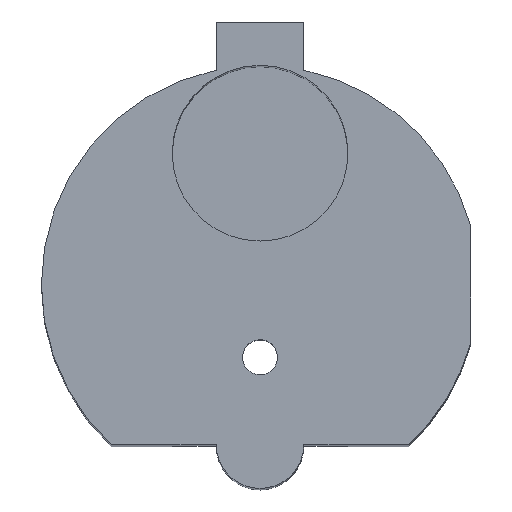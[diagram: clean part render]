
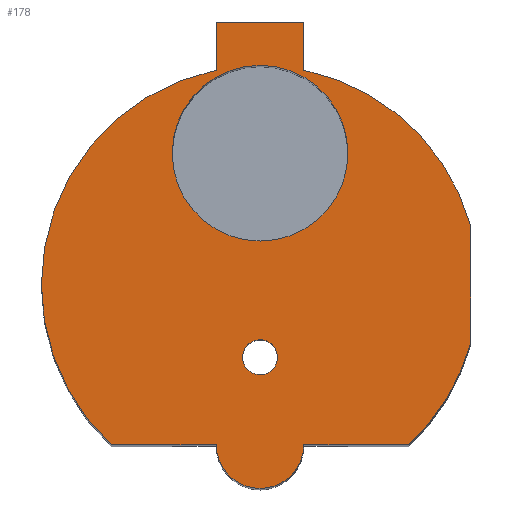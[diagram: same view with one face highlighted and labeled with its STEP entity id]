
A CAD part, top view. The second image highlights one B-rep face of the part: STEP entity #178.
In plain terms, the highlighted planar face has unit normal (0, 0, 1).
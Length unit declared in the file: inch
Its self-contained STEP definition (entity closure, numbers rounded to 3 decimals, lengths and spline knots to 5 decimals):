
#7 = AXIS2_PLACEMENT_3D ( 'NONE', #684, #1047, #1140 ) ;
#21 = AXIS2_PLACEMENT_3D ( 'NONE', #965, #514, #694 ) ;
#22 = VERTEX_POINT ( 'NONE', #44 ) ;
#27 = CARTESIAN_POINT ( 'NONE',  ( -0.15, 0.9, 2.9 ) ) ;
#42 = ORIENTED_EDGE ( 'NONE', *, *, #1071, .T. ) ;
#43 = CIRCLE ( 'NONE', #7, 0.75 ) ;
#44 = CARTESIAN_POINT ( 'NONE',  ( -0.30131, 0.45, 2.9 ) ) ;
#47 = ORIENTED_EDGE ( 'NONE', *, *, #1027, .F. ) ;
#55 = DIRECTION ( 'NONE',  ( 0., 0., 1. ) ) ;
#58 = PLANE ( 'NONE',  #457 ) ;
#68 = AXIS2_PLACEMENT_3D ( 'NONE', #913, #550, #823 ) ;
#70 = DIRECTION ( 'NONE',  ( 0., 1., 0. ) ) ;
#90 = ORIENTED_EDGE ( 'NONE', *, *, #865, .F. ) ;
#91 = VERTEX_POINT ( 'NONE', #329 ) ;
#103 = VERTEX_POINT ( 'NONE', #1134 ) ;
#105 = ORIENTED_EDGE ( 'NONE', *, *, #306, .F. ) ;
#108 = CARTESIAN_POINT ( 'NONE',  ( 0., -0.55, 2.9 ) ) ;
#112 = CIRCLE ( 'NONE', #620, 0.15 ) ;
#129 = AXIS2_PLACEMENT_3D ( 'NONE', #612, #55, #177 ) ;
#148 = DIRECTION ( 'NONE',  ( 0., -1., 0. ) ) ;
#177 = DIRECTION ( 'NONE',  ( 1., 0., 0. ) ) ;
#178 = ADVANCED_FACE ( 'NONE', ( #1092, #727, #943 ), #58, .T. ) ;
#201 = EDGE_CURVE ( 'NONE', #103, #91, #1144, .T. ) ;
#207 = VERTEX_POINT ( 'NONE', #982 ) ;
#211 = CARTESIAN_POINT ( 'NONE',  ( 0., 0.9, 2.9 ) ) ;
#223 = VERTEX_POINT ( 'NONE', #1039 ) ;
#229 = CARTESIAN_POINT ( 'NONE',  ( -0.15, 0., 2.9 ) ) ;
#235 = CARTESIAN_POINT ( 'NONE',  ( 0., -0.55, 2.9 ) ) ;
#255 = DIRECTION ( 'NONE',  ( 0., 0., -1. ) ) ;
#260 = EDGE_CURVE ( 'NONE', #561, #962, #885, .T. ) ;
#279 = VERTEX_POINT ( 'NONE', #798 ) ;
#304 = VERTEX_POINT ( 'NONE', #444 ) ;
#305 = CARTESIAN_POINT ( 'NONE',  ( -0.15, 0.73485, 2.9 ) ) ;
#306 = EDGE_CURVE ( 'NONE', #223, #22, #410, .T. ) ;
#310 = ORIENTED_EDGE ( 'NONE', *, *, #964, .T. ) ;
#312 = DIRECTION ( 'NONE',  ( 1., 0., 0. ) ) ;
#329 = CARTESIAN_POINT ( 'NONE',  ( -0.06, -0.25, 2.9 ) ) ;
#333 = LINE ( 'NONE', #563, #818 ) ;
#336 = LINE ( 'NONE', #526, #480 ) ;
#362 = DIRECTION ( 'NONE',  ( 1., 0., 0. ) ) ;
#374 = ORIENTED_EDGE ( 'NONE', *, *, #1106, .T. ) ;
#382 = CIRCLE ( 'NONE', #1146, 0.30131 ) ;
#410 = CIRCLE ( 'NONE', #961, 0.30131 ) ;
#424 = CIRCLE ( 'NONE', #1013, 0.06 ) ;
#425 = EDGE_CURVE ( 'NONE', #490, #207, #867, .T. ) ;
#440 = DIRECTION ( 'NONE',  ( 1., 0., 0. ) ) ;
#444 = CARTESIAN_POINT ( 'NONE',  ( -0.5099, -0.55, 2.9 ) ) ;
#446 = VECTOR ( 'NONE', #882, 39.37008 ) ;
#452 = CARTESIAN_POINT ( 'NONE',  ( 0., 0.45, 2.9 ) ) ;
#456 = DIRECTION ( 'NONE',  ( 0., 0., 1. ) ) ;
#457 = AXIS2_PLACEMENT_3D ( 'NONE', #975, #628, #440 ) ;
#478 = LINE ( 'NONE', #229, #1112 ) ;
#480 = VECTOR ( 'NONE', #70, 39.37008 ) ;
#490 = VERTEX_POINT ( 'NONE', #27 ) ;
#512 = DIRECTION ( 'NONE',  ( 1., 0., 0. ) ) ;
#514 = DIRECTION ( 'NONE',  ( 0., 0., 1. ) ) ;
#520 = LINE ( 'NONE', #108, #739 ) ;
#526 = CARTESIAN_POINT ( 'NONE',  ( 0.7222, 0., 2.9 ) ) ;
#533 = ORIENTED_EDGE ( 'NONE', *, *, #574, .T. ) ;
#539 = DIRECTION ( 'NONE',  ( 0., 0., 1. ) ) ;
#542 = CARTESIAN_POINT ( 'NONE',  ( 0.5099, -0.55, 2.9 ) ) ;
#550 = DIRECTION ( 'NONE',  ( 0., 0., -1. ) ) ;
#561 = VERTEX_POINT ( 'NONE', #542 ) ;
#563 = CARTESIAN_POINT ( 'NONE',  ( 0.15, 0., 2.9 ) ) ;
#573 = CARTESIAN_POINT ( 'NONE',  ( -0.15, -0.55, 2.9 ) ) ;
#574 = EDGE_CURVE ( 'NONE', #962, #747, #336, .T. ) ;
#576 = AXIS2_PLACEMENT_3D ( 'NONE', #980, #714, #721 ) ;
#592 = ORIENTED_EDGE ( 'NONE', *, *, #951, .T. ) ;
#594 = EDGE_CURVE ( 'NONE', #561, #920, #787, .T. ) ;
#612 = CARTESIAN_POINT ( 'NONE',  ( 0., 0., 2.9 ) ) ;
#620 = AXIS2_PLACEMENT_3D ( 'NONE', #235, #769, #512 ) ;
#628 = DIRECTION ( 'NONE',  ( 0., 0., 1. ) ) ;
#640 = VERTEX_POINT ( 'NONE', #1056 ) ;
#643 = CARTESIAN_POINT ( 'NONE',  ( 0.7222, 0.2023, 2.9 ) ) ;
#644 = ORIENTED_EDGE ( 'NONE', *, *, #738, .F. ) ;
#667 = ORIENTED_EDGE ( 'NONE', *, *, #425, .F. ) ;
#671 = EDGE_LOOP ( 'NONE', ( #1068, #791 ) ) ;
#684 = CARTESIAN_POINT ( 'NONE',  ( 0., 0., 2.9 ) ) ;
#694 = DIRECTION ( 'NONE',  ( 1., 0., 0. ) ) ;
#714 = DIRECTION ( 'NONE',  ( 0., 0., 1. ) ) ;
#721 = DIRECTION ( 'NONE',  ( 1., 0., 0. ) ) ;
#727 = FACE_BOUND ( 'NONE', #671, .T. ) ;
#738 = EDGE_CURVE ( 'NONE', #207, #279, #333, .T. ) ;
#739 = VECTOR ( 'NONE', #924, 39.37008 ) ;
#747 = VERTEX_POINT ( 'NONE', #643 ) ;
#768 = CIRCLE ( 'NONE', #576, 0.75 ) ;
#769 = DIRECTION ( 'NONE',  ( 0., 0., 1. ) ) ;
#787 = LINE ( 'NONE', #811, #446 ) ;
#791 = ORIENTED_EDGE ( 'NONE', *, *, #1097, .T. ) ;
#797 = ORIENTED_EDGE ( 'NONE', *, *, #994, .T. ) ;
#798 = CARTESIAN_POINT ( 'NONE',  ( 0.15, 0.73485, 2.9 ) ) ;
#811 = CARTESIAN_POINT ( 'NONE',  ( 0., -0.55, 2.9 ) ) ;
#818 = VECTOR ( 'NONE', #992, 39.37008 ) ;
#821 = VERTEX_POINT ( 'NONE', #305 ) ;
#823 = DIRECTION ( 'NONE',  ( 1., 0., 0. ) ) ;
#851 = VECTOR ( 'NONE', #312, 39.37008 ) ;
#865 = EDGE_CURVE ( 'NONE', #923, #304, #520, .T. ) ;
#867 = LINE ( 'NONE', #211, #851 ) ;
#882 = DIRECTION ( 'NONE',  ( -1., 0., 0. ) ) ;
#885 = CIRCLE ( 'NONE', #129, 0.75 ) ;
#896 = DIRECTION ( 'NONE',  ( 1., 0., 0. ) ) ;
#897 = CARTESIAN_POINT ( 'NONE',  ( 0., -0.25, 2.9 ) ) ;
#913 = CARTESIAN_POINT ( 'NONE',  ( 0., -0.25, 2.9 ) ) ;
#920 = VERTEX_POINT ( 'NONE', #1094 ) ;
#923 = VERTEX_POINT ( 'NONE', #573 ) ;
#924 = DIRECTION ( 'NONE',  ( -1., 0., 0. ) ) ;
#938 = EDGE_LOOP ( 'NONE', ( #1026, #533, #592, #644, #667, #310, #42, #797, #90, #374, #1038 ) ) ;
#943 = FACE_OUTER_BOUND ( 'NONE', #938, .T. ) ;
#948 = EDGE_LOOP ( 'NONE', ( #105, #47 ) ) ;
#951 = EDGE_CURVE ( 'NONE', #747, #279, #1141, .T. ) ;
#961 = AXIS2_PLACEMENT_3D ( 'NONE', #985, #456, #896 ) ;
#962 = VERTEX_POINT ( 'NONE', #1035 ) ;
#964 = EDGE_CURVE ( 'NONE', #490, #821, #478, .T. ) ;
#965 = CARTESIAN_POINT ( 'NONE',  ( 0., 0., 2.9 ) ) ;
#975 = CARTESIAN_POINT ( 'NONE',  ( 0., 0., 2.9 ) ) ;
#980 = CARTESIAN_POINT ( 'NONE',  ( 0., 0., 2.9 ) ) ;
#982 = CARTESIAN_POINT ( 'NONE',  ( 0.15, 0.9, 2.9 ) ) ;
#985 = CARTESIAN_POINT ( 'NONE',  ( 0., 0.45, 2.9 ) ) ;
#992 = DIRECTION ( 'NONE',  ( 0., -1., 0. ) ) ;
#994 = EDGE_CURVE ( 'NONE', #640, #304, #43, .T. ) ;
#1013 = AXIS2_PLACEMENT_3D ( 'NONE', #897, #255, #362 ) ;
#1026 = ORIENTED_EDGE ( 'NONE', *, *, #260, .T. ) ;
#1027 = EDGE_CURVE ( 'NONE', #22, #223, #382, .T. ) ;
#1035 = CARTESIAN_POINT ( 'NONE',  ( 0.7222, -0.2023, 2.9 ) ) ;
#1038 = ORIENTED_EDGE ( 'NONE', *, *, #594, .F. ) ;
#1039 = CARTESIAN_POINT ( 'NONE',  ( 0.30131, 0.45, 2.9 ) ) ;
#1047 = DIRECTION ( 'NONE',  ( 0., 0., 1. ) ) ;
#1056 = CARTESIAN_POINT ( 'NONE',  ( -0.75, 0., 2.9 ) ) ;
#1060 = DIRECTION ( 'NONE',  ( 1., 0., 0. ) ) ;
#1068 = ORIENTED_EDGE ( 'NONE', *, *, #201, .T. ) ;
#1071 = EDGE_CURVE ( 'NONE', #821, #640, #768, .T. ) ;
#1092 = FACE_BOUND ( 'NONE', #948, .T. ) ;
#1094 = CARTESIAN_POINT ( 'NONE',  ( 0.15, -0.55, 2.9 ) ) ;
#1097 = EDGE_CURVE ( 'NONE', #91, #103, #424, .T. ) ;
#1106 = EDGE_CURVE ( 'NONE', #923, #920, #112, .T. ) ;
#1112 = VECTOR ( 'NONE', #148, 39.37008 ) ;
#1134 = CARTESIAN_POINT ( 'NONE',  ( 0.06, -0.25, 2.9 ) ) ;
#1140 = DIRECTION ( 'NONE',  ( 1., 0., 0. ) ) ;
#1141 = CIRCLE ( 'NONE', #21, 0.75 ) ;
#1144 = CIRCLE ( 'NONE', #68, 0.06 ) ;
#1146 = AXIS2_PLACEMENT_3D ( 'NONE', #452, #539, #1060 ) ;
